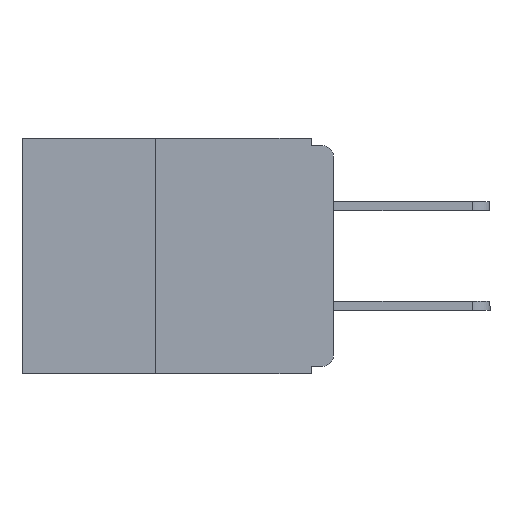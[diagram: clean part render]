
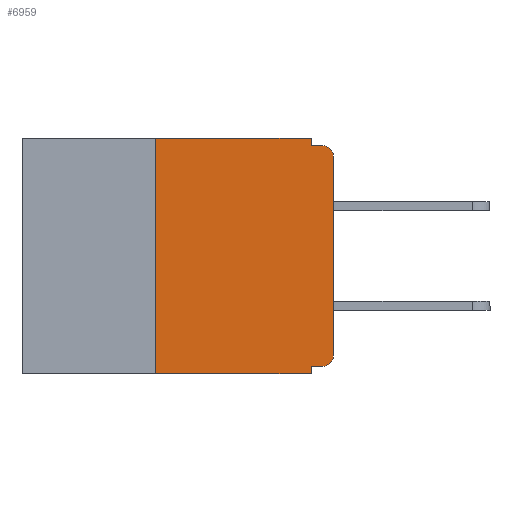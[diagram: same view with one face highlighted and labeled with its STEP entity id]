
A CAD part, left-side view. The second image highlights one B-rep face of the part: STEP entity #6959.
In plain terms, the highlighted planar face has unit normal (-1, 0, 0).
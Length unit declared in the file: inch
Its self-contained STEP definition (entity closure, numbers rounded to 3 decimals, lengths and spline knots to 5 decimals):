
#64 = CARTESIAN_POINT ( 'NONE',  ( 0., 0.031, -0.32 ) ) ;
#482 = AXIS2_PLACEMENT_3D ( 'NONE', #17944, #15221, #15065 ) ;
#1227 = ORIENTED_EDGE ( 'NONE', *, *, #10376, .F. ) ;
#1969 = CARTESIAN_POINT ( 'NONE',  ( 0., 0.031, 0. ) ) ;
#2031 = ORIENTED_EDGE ( 'NONE', *, *, #2134, .T. ) ;
#2134 = EDGE_CURVE ( 'NONE', #7690, #19091, #5301, .T. ) ;
#3826 = ORIENTED_EDGE ( 'NONE', *, *, #5204, .T. ) ;
#4343 = LINE ( 'NONE', #19960, #11068 ) ;
#5204 = EDGE_CURVE ( 'NONE', #6300, #7690, #15040, .T. ) ;
#5301 = LINE ( 'NONE', #14378, #19453 ) ;
#6300 = VERTEX_POINT ( 'NONE', #11024 ) ;
#6380 = LINE ( 'NONE', #1969, #19921 ) ;
#6606 = EDGE_CURVE ( 'NONE', #21684, #21123, #7487, .T. ) ;
#6617 = CARTESIAN_POINT ( 'NONE',  ( 0., 0.031, -0.01 ) ) ;
#6657 = VECTOR ( 'NONE', #10848, 39.37008 ) ;
#6918 = VERTEX_POINT ( 'NONE', #19088 ) ;
#6959 = ADVANCED_FACE ( 'NONE', ( #15844 ), #16181, .F. ) ;
#7487 = LINE ( 'NONE', #23602, #21538 ) ;
#7621 = VERTEX_POINT ( 'NONE', #6617 ) ;
#7690 = VERTEX_POINT ( 'NONE', #23263 ) ;
#8135 = DIRECTION ( 'NONE',  ( 0., 0., -1. ) ) ;
#8204 = DIRECTION ( 'NONE',  ( -1., 0., 0. ) ) ;
#8216 = CARTESIAN_POINT ( 'NONE',  ( 0., 0.015, -0.305 ) ) ;
#8990 = DIRECTION ( 'NONE',  ( 0., -1., 0. ) ) ;
#8993 = EDGE_CURVE ( 'NONE', #19091, #6918, #9748, .T. ) ;
#9010 = CARTESIAN_POINT ( 'NONE',  ( 0., 0.25, 0. ) ) ;
#9147 = EDGE_CURVE ( 'NONE', #21847, #21123, #20886, .T. ) ;
#9510 = DIRECTION ( 'NONE',  ( 0., -1., 0. ) ) ;
#9584 = CARTESIAN_POINT ( 'NONE',  ( 0., 0.25, -0.33 ) ) ;
#9659 = VERTEX_POINT ( 'NONE', #9010 ) ;
#9676 = LINE ( 'NONE', #9584, #23625 ) ;
#9748 = CIRCLE ( 'NONE', #12895, 0.015 ) ;
#9990 = CARTESIAN_POINT ( 'NONE',  ( 0., 0., -0.025 ) ) ;
#10376 = EDGE_CURVE ( 'NONE', #21847, #9659, #9676, .T. ) ;
#10848 = DIRECTION ( 'NONE',  ( 0., 1., 0. ) ) ;
#10883 = ORIENTED_EDGE ( 'NONE', *, *, #8993, .T. ) ;
#10886 = CARTESIAN_POINT ( 'NONE',  ( 0., 0.015, -0.025 ) ) ;
#11024 = CARTESIAN_POINT ( 'NONE',  ( 0., 0.015, -0.32 ) ) ;
#11068 = VECTOR ( 'NONE', #8990, 39.37008 ) ;
#11126 = ORIENTED_EDGE ( 'NONE', *, *, #6606, .F. ) ;
#11367 = DIRECTION ( 'NONE',  ( 0., 0., -1. ) ) ;
#11559 = ORIENTED_EDGE ( 'NONE', *, *, #14690, .F. ) ;
#11590 = EDGE_CURVE ( 'NONE', #18555, #7621, #6380, .T. ) ;
#11598 = LINE ( 'NONE', #19962, #6657 ) ;
#12022 = EDGE_LOOP ( 'NONE', ( #2031, #10883, #23401, #21542, #11559, #1227, #19607, #11126, #15140, #3826 ) ) ;
#12716 = EDGE_CURVE ( 'NONE', #6300, #21684, #11598, .T. ) ;
#12755 = DIRECTION ( 'NONE',  ( 0., 0., -1. ) ) ;
#12895 = AXIS2_PLACEMENT_3D ( 'NONE', #10886, #23598, #12755 ) ;
#12989 = AXIS2_PLACEMENT_3D ( 'NONE', #8216, #8204, #8135 ) ;
#13973 = DIRECTION ( 'NONE',  ( 0., 0., 1. ) ) ;
#14378 = CARTESIAN_POINT ( 'NONE',  ( 0., 0., 0. ) ) ;
#14690 = EDGE_CURVE ( 'NONE', #9659, #18555, #20937, .T. ) ;
#15040 = CIRCLE ( 'NONE', #12989, 0.015 ) ;
#15065 = DIRECTION ( 'NONE',  ( 0., 0., -1. ) ) ;
#15140 = ORIENTED_EDGE ( 'NONE', *, *, #12716, .F. ) ;
#15221 = DIRECTION ( 'NONE',  ( 1., 0., 0. ) ) ;
#15512 = VECTOR ( 'NONE', #15821, 39.37008 ) ;
#15821 = DIRECTION ( 'NONE',  ( 0., -1., 0. ) ) ;
#15844 = FACE_OUTER_BOUND ( 'NONE', #12022, .T. ) ;
#16142 = CARTESIAN_POINT ( 'NONE',  ( 0., 0.031, 0. ) ) ;
#16181 = PLANE ( 'NONE',  #482 ) ;
#16627 = VECTOR ( 'NONE', #9510, 39.37008 ) ;
#17457 = CARTESIAN_POINT ( 'NONE',  ( 0., 0.25, -0.33 ) ) ;
#17944 = CARTESIAN_POINT ( 'NONE',  ( 0., 0.437, 0. ) ) ;
#18555 = VERTEX_POINT ( 'NONE', #16142 ) ;
#19088 = CARTESIAN_POINT ( 'NONE',  ( 0., 0.015, -0.01 ) ) ;
#19091 = VERTEX_POINT ( 'NONE', #9990 ) ;
#19418 = CARTESIAN_POINT ( 'NONE',  ( 0., 0.437, 0. ) ) ;
#19453 = VECTOR ( 'NONE', #13973, 39.37008 ) ;
#19607 = ORIENTED_EDGE ( 'NONE', *, *, #9147, .T. ) ;
#19921 = VECTOR ( 'NONE', #11367, 39.37008 ) ;
#19960 = CARTESIAN_POINT ( 'NONE',  ( 0., 0., -0.01 ) ) ;
#19962 = CARTESIAN_POINT ( 'NONE',  ( 0., 0., -0.32 ) ) ;
#20456 = CARTESIAN_POINT ( 'NONE',  ( 0., 0.437, -0.33 ) ) ;
#20886 = LINE ( 'NONE', #20456, #16627 ) ;
#20937 = LINE ( 'NONE', #19418, #15512 ) ;
#21123 = VERTEX_POINT ( 'NONE', #23165 ) ;
#21237 = EDGE_CURVE ( 'NONE', #7621, #6918, #4343, .T. ) ;
#21538 = VECTOR ( 'NONE', #21911, 39.37008 ) ;
#21542 = ORIENTED_EDGE ( 'NONE', *, *, #11590, .F. ) ;
#21684 = VERTEX_POINT ( 'NONE', #64 ) ;
#21847 = VERTEX_POINT ( 'NONE', #17457 ) ;
#21911 = DIRECTION ( 'NONE',  ( 0., 0., -1. ) ) ;
#22396 = DIRECTION ( 'NONE',  ( 0., 0., 1. ) ) ;
#23165 = CARTESIAN_POINT ( 'NONE',  ( 0., 0.031, -0.33 ) ) ;
#23263 = CARTESIAN_POINT ( 'NONE',  ( 0., 0., -0.305 ) ) ;
#23401 = ORIENTED_EDGE ( 'NONE', *, *, #21237, .F. ) ;
#23598 = DIRECTION ( 'NONE',  ( -1., 0., 0. ) ) ;
#23602 = CARTESIAN_POINT ( 'NONE',  ( 0., 0.031, -0.33 ) ) ;
#23625 = VECTOR ( 'NONE', #22396, 39.37008 ) ;
